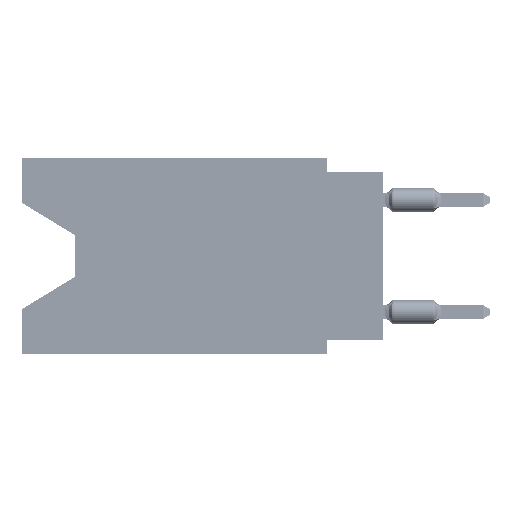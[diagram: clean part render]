
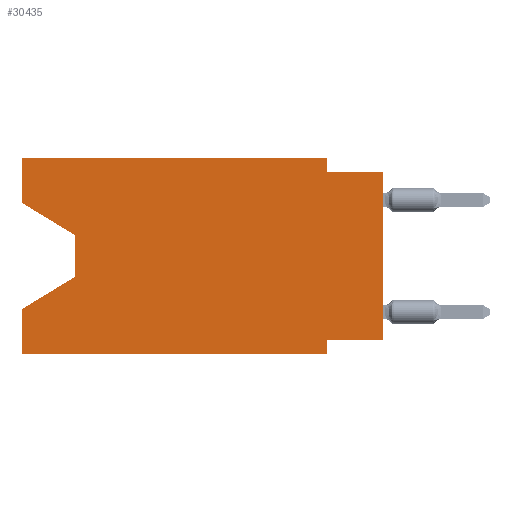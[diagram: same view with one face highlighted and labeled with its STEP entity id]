
A CAD part, left-side view. The second image highlights one B-rep face of the part: STEP entity #30435.
In plain terms, the highlighted planar face has unit normal (-1, 0, 0).
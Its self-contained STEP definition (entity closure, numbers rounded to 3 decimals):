
#14 = VECTOR ( 'NONE', #31169, 1000. ) ;
#991 = CARTESIAN_POINT ( 'NONE',  ( 0., 0., -8.255 ) ) ;
#1080 = LINE ( 'NONE', #80864, #24306 ) ;
#2552 = DIRECTION ( 'NONE',  ( 0., 0., 1. ) ) ;
#2622 = EDGE_CURVE ( 'NONE', #64132, #66382, #85174, .T. ) ;
#3997 = CARTESIAN_POINT ( 'NONE',  ( 0., 16.383, -2.038 ) ) ;
#6803 = PLANE ( 'NONE',  #69349 ) ;
#7508 = ORIENTED_EDGE ( 'NONE', *, *, #38951, .F. ) ;
#8841 = CARTESIAN_POINT ( 'NONE',  ( 0., 16.383, -8.89 ) ) ;
#9681 = LINE ( 'NONE', #24362, #68826 ) ;
#9727 = CARTESIAN_POINT ( 'NONE',  ( 0., 13.97, -3.505 ) ) ;
#9981 = EDGE_CURVE ( 'NONE', #69022, #64132, #37626, .T. ) ;
#10898 = CARTESIAN_POINT ( 'NONE',  ( 0., 13.97, -3.505 ) ) ;
#12799 = DIRECTION ( 'NONE',  ( 0., -1., 0. ) ) ;
#13433 = CARTESIAN_POINT ( 'NONE',  ( 0., 2.54, -8.89 ) ) ;
#13754 = VERTEX_POINT ( 'NONE', #60516 ) ;
#14808 = ORIENTED_EDGE ( 'NONE', *, *, #9981, .T. ) ;
#15941 = VERTEX_POINT ( 'NONE', #31279 ) ;
#16400 = VECTOR ( 'NONE', #30071, 1000. ) ;
#19468 = VERTEX_POINT ( 'NONE', #62589 ) ;
#20754 = CARTESIAN_POINT ( 'NONE',  ( 0., 2.54, -0.635 ) ) ;
#22825 = DIRECTION ( 'NONE',  ( 0., 0.855, -0.519 ) ) ;
#23139 = EDGE_CURVE ( 'NONE', #25110, #15941, #33349, .T. ) ;
#23188 = VECTOR ( 'NONE', #53436, 1000. ) ;
#23352 = EDGE_CURVE ( 'NONE', #63217, #37896, #9681, .T. ) ;
#24036 = LINE ( 'NONE', #3997, #14 ) ;
#24306 = VECTOR ( 'NONE', #33636, 1000. ) ;
#24318 = LINE ( 'NONE', #65303, #54476 ) ;
#24362 = CARTESIAN_POINT ( 'NONE',  ( 0., 16.383, 0. ) ) ;
#24893 = VERTEX_POINT ( 'NONE', #20754 ) ;
#25110 = VERTEX_POINT ( 'NONE', #991 ) ;
#26666 = DIRECTION ( 'NONE',  ( 0., 0., 1. ) ) ;
#27811 = ORIENTED_EDGE ( 'NONE', *, *, #69059, .T. ) ;
#28156 = DIRECTION ( 'NONE',  ( 0., 0., 1. ) ) ;
#28710 = ORIENTED_EDGE ( 'NONE', *, *, #36211, .T. ) ;
#30071 = DIRECTION ( 'NONE',  ( 0., 0., -1. ) ) ;
#30409 = ORIENTED_EDGE ( 'NONE', *, *, #47928, .F. ) ;
#30435 = ADVANCED_FACE ( 'NONE', ( #68710 ), #6803, .F. ) ;
#30566 = DIRECTION ( 'NONE',  ( 0., 0., -1. ) ) ;
#31169 = DIRECTION ( 'NONE',  ( 0., -0.855, -0.519 ) ) ;
#31279 = CARTESIAN_POINT ( 'NONE',  ( 0., 0., -0.635 ) ) ;
#32547 = CARTESIAN_POINT ( 'NONE',  ( 0., 2.54, -8.255 ) ) ;
#33349 = LINE ( 'NONE', #87684, #46443 ) ;
#33636 = DIRECTION ( 'NONE',  ( 0., 1., 0. ) ) ;
#34416 = VECTOR ( 'NONE', #2552, 1000. ) ;
#36211 = EDGE_CURVE ( 'NONE', #19468, #69022, #24036, .T. ) ;
#36248 = ORIENTED_EDGE ( 'NONE', *, *, #73856, .F. ) ;
#37626 = LINE ( 'NONE', #10898, #16400 ) ;
#37896 = VERTEX_POINT ( 'NONE', #45868 ) ;
#38951 = EDGE_CURVE ( 'NONE', #13754, #66382, #76689, .T. ) ;
#40187 = CARTESIAN_POINT ( 'NONE',  ( 0., 16.383, 0. ) ) ;
#40605 = DIRECTION ( 'NONE',  ( 0., 0., -1. ) ) ;
#40668 = DIRECTION ( 'NONE',  ( 1., 0., 0. ) ) ;
#40839 = EDGE_LOOP ( 'NONE', ( #28710, #14808, #63457, #7508, #27811, #36248, #49863, #57640, #87274, #86744, #73586, #30409 ) ) ;
#43893 = VECTOR ( 'NONE', #12799, 1000. ) ;
#44067 = CARTESIAN_POINT ( 'NONE',  ( 0., 2.54, -8.89 ) ) ;
#45868 = CARTESIAN_POINT ( 'NONE',  ( 0., 2.54, 0. ) ) ;
#46443 = VECTOR ( 'NONE', #26666, 1000. ) ;
#47658 = VERTEX_POINT ( 'NONE', #44067 ) ;
#47928 = EDGE_CURVE ( 'NONE', #19468, #63217, #55142, .T. ) ;
#49343 = CARTESIAN_POINT ( 'NONE',  ( 0., 16.383, 0. ) ) ;
#49863 = ORIENTED_EDGE ( 'NONE', *, *, #65724, .F. ) ;
#52989 = VECTOR ( 'NONE', #28156, 1000. ) ;
#53427 = VERTEX_POINT ( 'NONE', #32547 ) ;
#53436 = DIRECTION ( 'NONE',  ( 0., -1., 0. ) ) ;
#54476 = VECTOR ( 'NONE', #30566, 1000. ) ;
#55142 = LINE ( 'NONE', #49343, #34416 ) ;
#55966 = EDGE_CURVE ( 'NONE', #37896, #24893, #24318, .T. ) ;
#57640 = ORIENTED_EDGE ( 'NONE', *, *, #23139, .T. ) ;
#58661 = DIRECTION ( 'NONE',  ( 0., -1., 0. ) ) ;
#59250 = CARTESIAN_POINT ( 'NONE',  ( 0., 0., -0.635 ) ) ;
#59901 = VECTOR ( 'NONE', #22825, 1000. ) ;
#60516 = CARTESIAN_POINT ( 'NONE',  ( 0., 16.383, -8.89 ) ) ;
#60726 = CARTESIAN_POINT ( 'NONE',  ( 0., 16.383, 0. ) ) ;
#62589 = CARTESIAN_POINT ( 'NONE',  ( 0., 16.383, -2.038 ) ) ;
#62948 = VECTOR ( 'NONE', #40605, 1000. ) ;
#63217 = VERTEX_POINT ( 'NONE', #40187 ) ;
#63330 = CARTESIAN_POINT ( 'NONE',  ( 0., 16.383, 0. ) ) ;
#63457 = ORIENTED_EDGE ( 'NONE', *, *, #2622, .T. ) ;
#64132 = VERTEX_POINT ( 'NONE', #70672 ) ;
#65303 = CARTESIAN_POINT ( 'NONE',  ( 0., 2.54, 0. ) ) ;
#65724 = EDGE_CURVE ( 'NONE', #25110, #53427, #1080, .T. ) ;
#66382 = VERTEX_POINT ( 'NONE', #79649 ) ;
#68710 = FACE_OUTER_BOUND ( 'NONE', #40839, .T. ) ;
#68826 = VECTOR ( 'NONE', #58661, 1000. ) ;
#69022 = VERTEX_POINT ( 'NONE', #9727 ) ;
#69059 = EDGE_CURVE ( 'NONE', #13754, #47658, #69873, .T. ) ;
#69349 = AXIS2_PLACEMENT_3D ( 'NONE', #60726, #40668, #74519 ) ;
#69873 = LINE ( 'NONE', #8841, #43893 ) ;
#70672 = CARTESIAN_POINT ( 'NONE',  ( 0., 13.97, -5.385 ) ) ;
#71373 = CARTESIAN_POINT ( 'NONE',  ( 0., 13.97, -5.385 ) ) ;
#73586 = ORIENTED_EDGE ( 'NONE', *, *, #23352, .F. ) ;
#73856 = EDGE_CURVE ( 'NONE', #53427, #47658, #80272, .T. ) ;
#74519 = DIRECTION ( 'NONE',  ( 0., 0., -1. ) ) ;
#75623 = EDGE_CURVE ( 'NONE', #24893, #15941, #81050, .T. ) ;
#76689 = LINE ( 'NONE', #63330, #52989 ) ;
#79649 = CARTESIAN_POINT ( 'NONE',  ( 0., 16.383, -6.852 ) ) ;
#80272 = LINE ( 'NONE', #13433, #62948 ) ;
#80864 = CARTESIAN_POINT ( 'NONE',  ( 0., 0., -8.255 ) ) ;
#81050 = LINE ( 'NONE', #59250, #23188 ) ;
#85174 = LINE ( 'NONE', #71373, #59901 ) ;
#86744 = ORIENTED_EDGE ( 'NONE', *, *, #55966, .F. ) ;
#87274 = ORIENTED_EDGE ( 'NONE', *, *, #75623, .F. ) ;
#87684 = CARTESIAN_POINT ( 'NONE',  ( 0., 0., 0. ) ) ;
